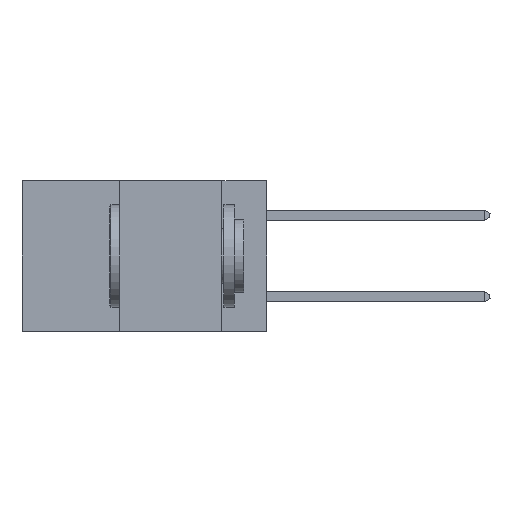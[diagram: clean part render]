
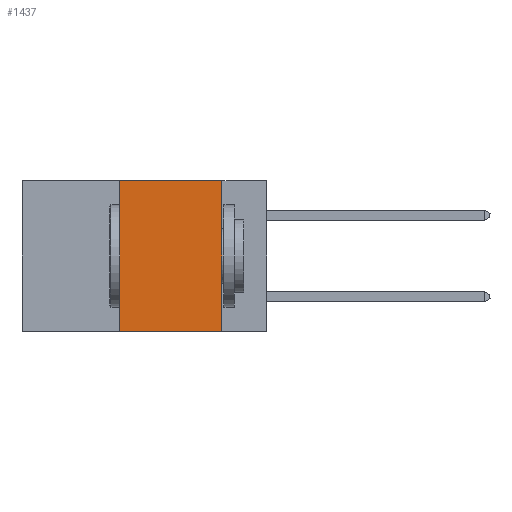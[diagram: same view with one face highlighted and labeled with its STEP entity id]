
A CAD part, left-side view. The second image highlights one B-rep face of the part: STEP entity #1437.
In plain terms, the highlighted planar face has unit normal (-1, 0, 0).
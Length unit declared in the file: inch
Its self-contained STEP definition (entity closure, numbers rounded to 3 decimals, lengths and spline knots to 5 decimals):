
#966 = DIRECTION ( 'NONE',  ( 0., -1., 0. ) ) ;
#1437 = ADVANCED_FACE ( 'NONE', ( #16337 ), #14233, .F. ) ;
#3246 = VECTOR ( 'NONE', #26369, 39.37008 ) ;
#3407 = CARTESIAN_POINT ( 'NONE',  ( 0., 0.6, -0.37 ) ) ;
#4598 = ORIENTED_EDGE ( 'NONE', *, *, #17956, .T. ) ;
#4772 = CARTESIAN_POINT ( 'NONE',  ( 0., 0.11, 0. ) ) ;
#5571 = VERTEX_POINT ( 'NONE', #22399 ) ;
#6530 = DIRECTION ( 'NONE',  ( 1., 0., 0. ) ) ;
#6858 = CARTESIAN_POINT ( 'NONE',  ( 0., 0.11, -0.37 ) ) ;
#8612 = VERTEX_POINT ( 'NONE', #4772 ) ;
#9183 = CARTESIAN_POINT ( 'NONE',  ( 0., 0.6, 0. ) ) ;
#10996 = ORIENTED_EDGE ( 'NONE', *, *, #22902, .F. ) ;
#11582 = DIRECTION ( 'NONE',  ( 0., 0., -1. ) ) ;
#11770 = CARTESIAN_POINT ( 'NONE',  ( 0., 0.11, 0. ) ) ;
#12491 = LINE ( 'NONE', #11770, #30883 ) ;
#14108 = AXIS2_PLACEMENT_3D ( 'NONE', #19256, #6530, #11582 ) ;
#14233 = PLANE ( 'NONE',  #14108 ) ;
#15576 = ORIENTED_EDGE ( 'NONE', *, *, #20394, .F. ) ;
#15702 = CARTESIAN_POINT ( 'NONE',  ( 0., 0.36, 0. ) ) ;
#16337 = FACE_OUTER_BOUND ( 'NONE', #27230, .T. ) ;
#16765 = VECTOR ( 'NONE', #26069, 39.37008 ) ;
#16795 = DIRECTION ( 'NONE',  ( 0., 0., -1. ) ) ;
#17543 = LINE ( 'NONE', #15702, #16765 ) ;
#17956 = EDGE_CURVE ( 'NONE', #5571, #30258, #18854, .T. ) ;
#18854 = LINE ( 'NONE', #3407, #30978 ) ;
#19256 = CARTESIAN_POINT ( 'NONE',  ( 0., 0.6, 0. ) ) ;
#20394 = EDGE_CURVE ( 'NONE', #5571, #26713, #17543, .T. ) ;
#21460 = CARTESIAN_POINT ( 'NONE',  ( 0., 0.36, 0. ) ) ;
#22399 = CARTESIAN_POINT ( 'NONE',  ( 0., 0.36, -0.37 ) ) ;
#22902 = EDGE_CURVE ( 'NONE', #26713, #8612, #27918, .T. ) ;
#26069 = DIRECTION ( 'NONE',  ( 0., 0., 1. ) ) ;
#26369 = DIRECTION ( 'NONE',  ( 0., -1., 0. ) ) ;
#26713 = VERTEX_POINT ( 'NONE', #21460 ) ;
#27230 = EDGE_LOOP ( 'NONE', ( #32235, #10996, #15576, #4598 ) ) ;
#27918 = LINE ( 'NONE', #9183, #3246 ) ;
#30258 = VERTEX_POINT ( 'NONE', #6858 ) ;
#30883 = VECTOR ( 'NONE', #16795, 39.37008 ) ;
#30934 = EDGE_CURVE ( 'NONE', #8612, #30258, #12491, .T. ) ;
#30978 = VECTOR ( 'NONE', #966, 39.37008 ) ;
#32235 = ORIENTED_EDGE ( 'NONE', *, *, #30934, .F. ) ;
